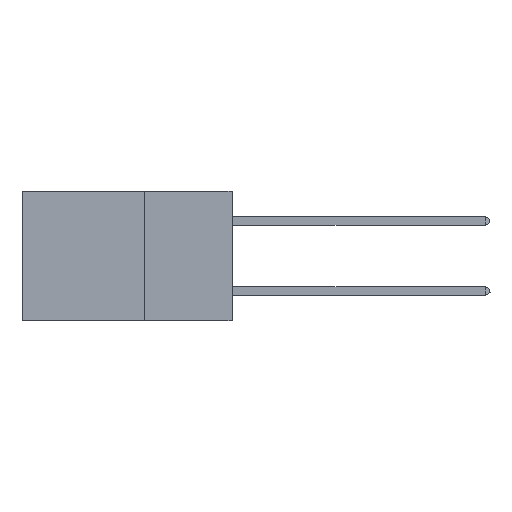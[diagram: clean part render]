
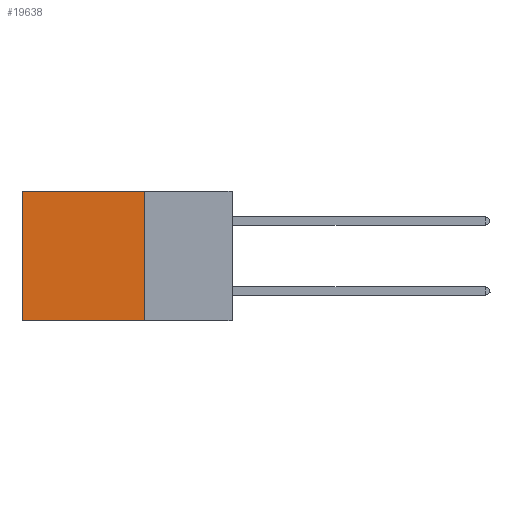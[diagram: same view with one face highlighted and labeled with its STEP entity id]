
A CAD part, left-side view. The second image highlights one B-rep face of the part: STEP entity #19638.
In plain terms, the highlighted planar face has unit normal (-1, 0, 0).
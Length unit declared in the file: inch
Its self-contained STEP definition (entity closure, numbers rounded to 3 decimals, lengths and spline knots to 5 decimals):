
#29 = VECTOR ( 'NONE', #13286, 39.37008 ) ;
#772 = CARTESIAN_POINT ( 'NONE',  ( 0.2875, 0.6, -0.37 ) ) ;
#888 = DIRECTION ( 'NONE',  ( 0., 0., -1. ) ) ;
#3733 = DIRECTION ( 'NONE',  ( 0., 0., -1. ) ) ;
#5324 = FACE_OUTER_BOUND ( 'NONE', #17496, .T. ) ;
#5333 = CARTESIAN_POINT ( 'NONE',  ( 0.2875, 0.6, 0. ) ) ;
#5933 = LINE ( 'NONE', #19558, #14846 ) ;
#6171 = ORIENTED_EDGE ( 'NONE', *, *, #6226, .T. ) ;
#6226 = EDGE_CURVE ( 'NONE', #15631, #10702, #22099, .T. ) ;
#6329 = CARTESIAN_POINT ( 'NONE',  ( 0.2875, 0.25, -0.37 ) ) ;
#7786 = VECTOR ( 'NONE', #20885, 39.37008 ) ;
#7822 = VERTEX_POINT ( 'NONE', #16950 ) ;
#9226 = VERTEX_POINT ( 'NONE', #772 ) ;
#9537 = PLANE ( 'NONE',  #17831 ) ;
#9692 = CARTESIAN_POINT ( 'NONE',  ( 0.2875, 0.25, 0. ) ) ;
#9736 = CARTESIAN_POINT ( 'NONE',  ( 0.2875, 0.25, 0. ) ) ;
#10235 = EDGE_CURVE ( 'NONE', #7822, #9226, #12757, .T. ) ;
#10702 = VERTEX_POINT ( 'NONE', #16543 ) ;
#11028 = EDGE_CURVE ( 'NONE', #15631, #7822, #5933, .T. ) ;
#11317 = LINE ( 'NONE', #5333, #20204 ) ;
#11439 = DIRECTION ( 'NONE',  ( 1., 0., 0. ) ) ;
#12757 = LINE ( 'NONE', #6329, #29 ) ;
#12769 = DIRECTION ( 'NONE',  ( 0., 0., -1. ) ) ;
#13286 = DIRECTION ( 'NONE',  ( 0., 1., 0. ) ) ;
#14531 = ORIENTED_EDGE ( 'NONE', *, *, #11028, .F. ) ;
#14846 = VECTOR ( 'NONE', #12769, 39.37008 ) ;
#15631 = VERTEX_POINT ( 'NONE', #9736 ) ;
#15634 = CARTESIAN_POINT ( 'NONE',  ( 0.2875, 0.25, 0. ) ) ;
#16543 = CARTESIAN_POINT ( 'NONE',  ( 0.2875, 0.6, 0. ) ) ;
#16950 = CARTESIAN_POINT ( 'NONE',  ( 0.2875, 0.25, -0.37 ) ) ;
#17496 = EDGE_LOOP ( 'NONE', ( #20908, #18848, #14531, #6171 ) ) ;
#17831 = AXIS2_PLACEMENT_3D ( 'NONE', #9692, #11439, #888 ) ;
#18318 = EDGE_CURVE ( 'NONE', #10702, #9226, #11317, .T. ) ;
#18848 = ORIENTED_EDGE ( 'NONE', *, *, #10235, .F. ) ;
#19558 = CARTESIAN_POINT ( 'NONE',  ( 0.2875, 0.25, 0. ) ) ;
#19638 = ADVANCED_FACE ( 'NONE', ( #5324 ), #9537, .F. ) ;
#20204 = VECTOR ( 'NONE', #3733, 39.37008 ) ;
#20885 = DIRECTION ( 'NONE',  ( 0., 1., 0. ) ) ;
#20908 = ORIENTED_EDGE ( 'NONE', *, *, #18318, .T. ) ;
#22099 = LINE ( 'NONE', #15634, #7786 ) ;
